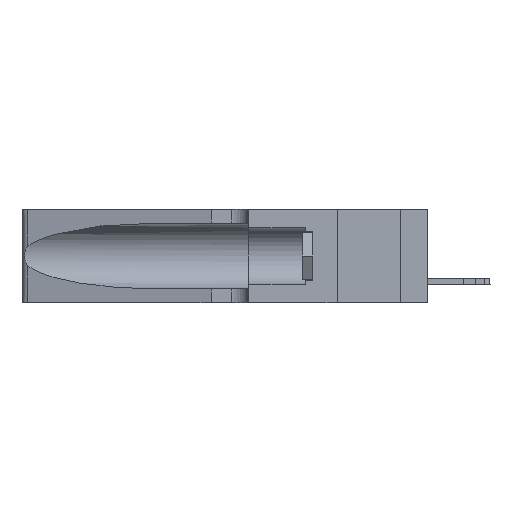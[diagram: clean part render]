
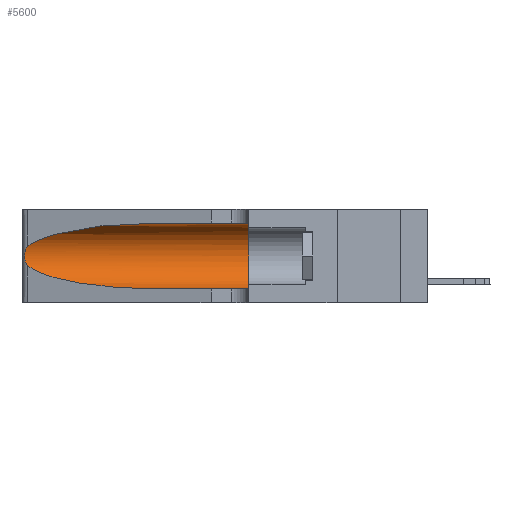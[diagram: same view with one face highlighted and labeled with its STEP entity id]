
A CAD part, left-side view. The second image highlights one B-rep face of the part: STEP entity #5600.
In plain terms, the highlighted cylindrical face has radius 3.308 mm (diameter 6.617 mm), a partial arc.
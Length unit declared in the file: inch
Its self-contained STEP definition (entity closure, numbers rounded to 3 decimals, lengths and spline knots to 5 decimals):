
#228 = CYLINDRICAL_SURFACE ( 'NONE', #26651, 0.13025 ) ;
#304 = CARTESIAN_POINT ( 'NONE',  ( 0.1305, 0.35, 0.185 ) ) ;
#393 = DIRECTION ( 'NONE',  ( 0., -1., 0. ) ) ;
#545 = EDGE_LOOP ( 'NONE', ( #11390, #3605, #5996, #16025, #26413, #20968 ) ) ;
#1063 = AXIS2_PLACEMENT_3D ( 'NONE', #304, #20276, #14313 ) ;
#1502 = LINE ( 'NONE', #29787, #23509 ) ;
#1903 = CARTESIAN_POINT ( 'NONE',  ( 0.25555, 1.22994, 0.2215 ) ) ;
#2009 = CARTESIAN_POINT ( 'NONE',  ( 0.25789, 1.23486, 0.15765 ) ) ;
#2465 = DIRECTION ( 'NONE',  ( 0., 0., -1. ) ) ;
#3167 = CARTESIAN_POINT ( 'NONE',  ( 0.25487, 1.22718, 0.22369 ) ) ;
#3412 = CARTESIAN_POINT ( 'NONE',  ( 0.1305, 0.72297, 0.31525 ) ) ;
#3446 =( BOUNDED_CURVE ( )  B_SPLINE_CURVE ( 3, ( #3412, #5613, #8316, #3167 ),
 .UNSPECIFIED., .F., .T. ) 
 B_SPLINE_CURVE_WITH_KNOTS ( ( 4, 4 ),
 ( 1.5708, 2.84003 ),
 .UNSPECIFIED. ) 
 CURVE ( )  GEOMETRIC_REPRESENTATION_ITEM ( )  RATIONAL_B_SPLINE_CURVE ( ( 1., 0.87, 0.87, 1. ) ) 
 REPRESENTATION_ITEM ( '' )  );
#3605 = ORIENTED_EDGE ( 'NONE', *, *, #4519, .T. ) ;
#4519 = EDGE_CURVE ( 'NONE', #22801, #22037, #7929, .T. ) ;
#4654 = CARTESIAN_POINT ( 'NONE',  ( 0.26018, 1.23835, 0.19895 ) ) ;
#5206 = CARTESIAN_POINT ( 'NONE',  ( 0.1305, 0.35, 0.05475 ) ) ;
#5600 = ADVANCED_FACE ( 'NONE', ( #19148 ), #228, .F. ) ;
#5613 = CARTESIAN_POINT ( 'NONE',  ( 0.18966, 0.96281, 0.31525 ) ) ;
#5824 = CARTESIAN_POINT ( 'NONE',  ( 0.25487, 1.22718, 0.14631 ) ) ;
#5996 = ORIENTED_EDGE ( 'NONE', *, *, #19805, .T. ) ;
#7187 = CARTESIAN_POINT ( 'NONE',  ( 0.25555, 1.22993, 0.14849 ) ) ;
#7864 = CARTESIAN_POINT ( 'NONE',  ( 0.2373, 1.15595, 0.08982 ) ) ;
#7929 = B_SPLINE_CURVE_WITH_KNOTS ( 'NONE', 3,
 ( #30259, #1903, #14836, #32619, #24645, #4654, #32408, #17408, #17517, #19886, #2009, #19653, #7187, #22561 ),
 .UNSPECIFIED., .F., .F.,
 ( 4, 2, 2, 2, 2, 2, 4 ),
 ( 0., 0.00027, 0.00053, 0.00107, 0.0016, 0.00187, 0.00214 ),
 .UNSPECIFIED. ) ;
#8316 = CARTESIAN_POINT ( 'NONE',  ( 0.2373, 1.15595, 0.28018 ) ) ;
#8706 = CIRCLE ( 'NONE', #1063, 0.13025 ) ;
#9156 = CARTESIAN_POINT ( 'NONE',  ( 0.25487, 1.22718, 0.14631 ) ) ;
#10979 = CARTESIAN_POINT ( 'NONE',  ( 0.1305, 1.61858, 0.31525 ) ) ;
#11390 = ORIENTED_EDGE ( 'NONE', *, *, #17959, .T. ) ;
#12088 = VERTEX_POINT ( 'NONE', #5206 ) ;
#13231 = EDGE_CURVE ( 'NONE', #26866, #12088, #1502, .T. ) ;
#13308 = EDGE_CURVE ( 'NONE', #17009, #12088, #8706, .T. ) ;
#13350 = CARTESIAN_POINT ( 'NONE',  ( 0.1305, 0.35, 0.31525 ) ) ;
#14313 = DIRECTION ( 'NONE',  ( 0., 0., 1. ) ) ;
#14836 = CARTESIAN_POINT ( 'NONE',  ( 0.25639, 1.23184, 0.21858 ) ) ;
#16025 = ORIENTED_EDGE ( 'NONE', *, *, #13231, .T. ) ;
#16353 = VECTOR ( 'NONE', #393, 39.37008 ) ;
#16802 = CARTESIAN_POINT ( 'NONE',  ( 0.1305, 0.72297, 0.05475 ) ) ;
#17009 = VERTEX_POINT ( 'NONE', #13350 ) ;
#17408 = CARTESIAN_POINT ( 'NONE',  ( 0.26075, 1.23896, 0.178 ) ) ;
#17517 = CARTESIAN_POINT ( 'NONE',  ( 0.26017, 1.23833, 0.17102 ) ) ;
#17655 = DIRECTION ( 'NONE',  ( 0., -1., 0. ) ) ;
#17959 = EDGE_CURVE ( 'NONE', #21977, #22801, #3446, .T. ) ;
#18552 = CARTESIAN_POINT ( 'NONE',  ( 0.25487, 1.22718, 0.22369 ) ) ;
#18756 = LINE ( 'NONE', #10979, #16353 ) ;
#19148 = FACE_OUTER_BOUND ( 'NONE', #545, .T. ) ;
#19653 = CARTESIAN_POINT ( 'NONE',  ( 0.25639, 1.23186, 0.15144 ) ) ;
#19805 = EDGE_CURVE ( 'NONE', #22037, #26866, #21763, .T. ) ;
#19886 = CARTESIAN_POINT ( 'NONE',  ( 0.25856, 1.23593, 0.16098 ) ) ;
#20276 = DIRECTION ( 'NONE',  ( 0., 1., 0. ) ) ;
#20968 = ORIENTED_EDGE ( 'NONE', *, *, #24559, .F. ) ;
#21763 =( BOUNDED_CURVE ( )  B_SPLINE_CURVE ( 3, ( #5824, #7864, #28912, #26657 ),
 .UNSPECIFIED., .F., .T. ) 
 B_SPLINE_CURVE_WITH_KNOTS ( ( 4, 4 ),
 ( 3.44316, 4.71239 ),
 .UNSPECIFIED. ) 
 CURVE ( )  GEOMETRIC_REPRESENTATION_ITEM ( )  RATIONAL_B_SPLINE_CURVE ( ( 1., 0.87, 0.87, 1. ) ) 
 REPRESENTATION_ITEM ( '' )  );
#21977 = VERTEX_POINT ( 'NONE', #32024 ) ;
#22037 = VERTEX_POINT ( 'NONE', #9156 ) ;
#22561 = CARTESIAN_POINT ( 'NONE',  ( 0.25487, 1.22718, 0.14631 ) ) ;
#22801 = VERTEX_POINT ( 'NONE', #18552 ) ;
#23509 = VECTOR ( 'NONE', #24159, 39.37008 ) ;
#24159 = DIRECTION ( 'NONE',  ( 0., -1., 0. ) ) ;
#24559 = EDGE_CURVE ( 'NONE', #21977, #17009, #18756, .T. ) ;
#24645 = CARTESIAN_POINT ( 'NONE',  ( 0.25854, 1.2359, 0.20912 ) ) ;
#26413 = ORIENTED_EDGE ( 'NONE', *, *, #13308, .F. ) ;
#26651 = AXIS2_PLACEMENT_3D ( 'NONE', #27993, #17655, #2465 ) ;
#26657 = CARTESIAN_POINT ( 'NONE',  ( 0.1305, 0.72297, 0.05475 ) ) ;
#26866 = VERTEX_POINT ( 'NONE', #16802 ) ;
#27993 = CARTESIAN_POINT ( 'NONE',  ( 0.1305, 1.61858, 0.185 ) ) ;
#28912 = CARTESIAN_POINT ( 'NONE',  ( 0.18966, 0.96281, 0.05475 ) ) ;
#29787 = CARTESIAN_POINT ( 'NONE',  ( 0.1305, 1.61858, 0.05475 ) ) ;
#30259 = CARTESIAN_POINT ( 'NONE',  ( 0.25487, 1.22718, 0.22369 ) ) ;
#32024 = CARTESIAN_POINT ( 'NONE',  ( 0.1305, 0.72297, 0.31525 ) ) ;
#32408 = CARTESIAN_POINT ( 'NONE',  ( 0.26075, 1.23896, 0.19203 ) ) ;
#32619 = CARTESIAN_POINT ( 'NONE',  ( 0.25787, 1.23484, 0.2124 ) ) ;
